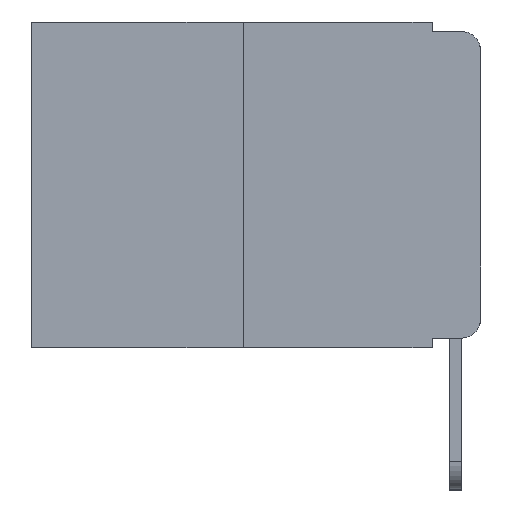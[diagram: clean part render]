
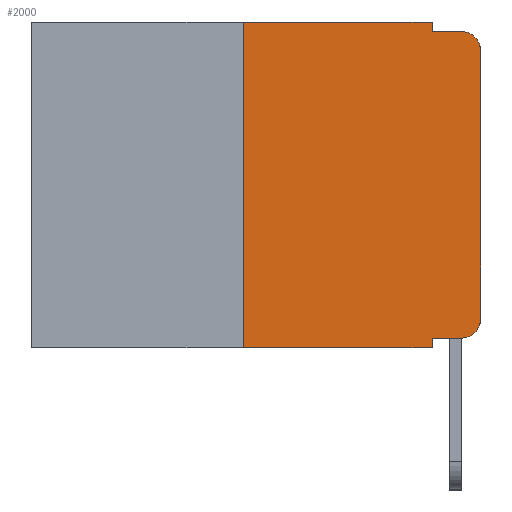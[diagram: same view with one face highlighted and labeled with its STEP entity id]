
A CAD part, left-side view. The second image highlights one B-rep face of the part: STEP entity #2000.
In plain terms, the highlighted planar face has unit normal (-1, 0, 0).
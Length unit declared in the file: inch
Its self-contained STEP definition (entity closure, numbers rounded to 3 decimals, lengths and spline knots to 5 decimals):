
#30 = FACE_OUTER_BOUND ( 'NONE', #903, .T. ) ;
#32 = EDGE_CURVE ( 'NONE', #7247, #2983, #8644, .T. ) ;
#239 = LINE ( 'NONE', #11429, #5632 ) ;
#250 = AXIS2_PLACEMENT_3D ( 'NONE', #5185, #4785, #8455 ) ;
#743 = CARTESIAN_POINT ( 'NONE',  ( 0., 0.051, 0. ) ) ;
#797 = CARTESIAN_POINT ( 'NONE',  ( 0., 0.25, 0. ) ) ;
#903 = EDGE_LOOP ( 'NONE', ( #8469, #4815, #4759, #4670, #4480, #4424, #4358, #4037, #3895, #3824 ) ) ;
#1348 = CARTESIAN_POINT ( 'NONE',  ( 0., 0., -0.03 ) ) ;
#1365 = CARTESIAN_POINT ( 'NONE',  ( 0., 0.051, -0.343 ) ) ;
#1489 = EDGE_CURVE ( 'NONE', #8368, #1525, #239, .T. ) ;
#1525 = VERTEX_POINT ( 'NONE', #1365 ) ;
#1577 = EDGE_CURVE ( 'NONE', #8368, #5704, #2273, .T. ) ;
#1839 = EDGE_CURVE ( 'NONE', #5704, #11722, #10260, .T. ) ;
#1909 = VECTOR ( 'NONE', #2441, 39.37008 ) ;
#1931 = DIRECTION ( 'NONE',  ( 0., 0., 1. ) ) ;
#1970 = CARTESIAN_POINT ( 'NONE',  ( 0., 0.051, -0.333 ) ) ;
#2000 = ADVANCED_FACE ( 'NONE', ( #30 ), #6648, .F. ) ;
#2273 = LINE ( 'NONE', #1970, #9714 ) ;
#2441 = DIRECTION ( 'NONE',  ( 0., -1., 0. ) ) ;
#2983 = VERTEX_POINT ( 'NONE', #10636 ) ;
#3414 = CARTESIAN_POINT ( 'NONE',  ( 0., 0.02, -0.313 ) ) ;
#3684 = CIRCLE ( 'NONE', #7859, 0.02 ) ;
#3748 = DIRECTION ( 'NONE',  ( 0., 0., 1. ) ) ;
#3788 = CARTESIAN_POINT ( 'NONE',  ( 0., 0.02, -0.03 ) ) ;
#3824 = ORIENTED_EDGE ( 'NONE', *, *, #1839, .T. ) ;
#3895 = ORIENTED_EDGE ( 'NONE', *, *, #1577, .T. ) ;
#4037 = ORIENTED_EDGE ( 'NONE', *, *, #1489, .F. ) ;
#4207 = VECTOR ( 'NONE', #6423, 39.37008 ) ;
#4358 = ORIENTED_EDGE ( 'NONE', *, *, #11394, .T. ) ;
#4424 = ORIENTED_EDGE ( 'NONE', *, *, #32, .F. ) ;
#4480 = ORIENTED_EDGE ( 'NONE', *, *, #7723, .F. ) ;
#4621 = VERTEX_POINT ( 'NONE', #8294 ) ;
#4670 = ORIENTED_EDGE ( 'NONE', *, *, #11001, .F. ) ;
#4698 = LINE ( 'NONE', #9266, #1909 ) ;
#4759 = ORIENTED_EDGE ( 'NONE', *, *, #10922, .F. ) ;
#4778 = DIRECTION ( 'NONE',  ( 0., 0., -1. ) ) ;
#4785 = DIRECTION ( 'NONE',  ( 1., 0., 0. ) ) ;
#4815 = ORIENTED_EDGE ( 'NONE', *, *, #10865, .T. ) ;
#4828 = CARTESIAN_POINT ( 'NONE',  ( 0., 0.051, -0.01 ) ) ;
#4966 = VERTEX_POINT ( 'NONE', #11161 ) ;
#5185 = CARTESIAN_POINT ( 'NONE',  ( 0., 0.473, 0. ) ) ;
#5580 = AXIS2_PLACEMENT_3D ( 'NONE', #3414, #6360, #10184 ) ;
#5632 = VECTOR ( 'NONE', #8456, 39.37008 ) ;
#5704 = VERTEX_POINT ( 'NONE', #12509 ) ;
#6018 = LINE ( 'NONE', #4828, #10855 ) ;
#6133 = VECTOR ( 'NONE', #1931, 39.37008 ) ;
#6360 = DIRECTION ( 'NONE',  ( -1., 0., 0. ) ) ;
#6423 = DIRECTION ( 'NONE',  ( 0., -1., 0. ) ) ;
#6583 = LINE ( 'NONE', #10343, #11357 ) ;
#6648 = PLANE ( 'NONE',  #250 ) ;
#6775 = LINE ( 'NONE', #7334, #4207 ) ;
#7021 = DIRECTION ( 'NONE',  ( 0., 0., -1. ) ) ;
#7247 = VERTEX_POINT ( 'NONE', #11215 ) ;
#7334 = CARTESIAN_POINT ( 'NONE',  ( 0., 0.473, -0.343 ) ) ;
#7723 = EDGE_CURVE ( 'NONE', #2983, #4621, #4698, .T. ) ;
#7739 = VERTEX_POINT ( 'NONE', #1348 ) ;
#7859 = AXIS2_PLACEMENT_3D ( 'NONE', #3788, #10387, #4778 ) ;
#7893 = CARTESIAN_POINT ( 'NONE',  ( 0., 0., -0.313 ) ) ;
#8294 = CARTESIAN_POINT ( 'NONE',  ( 0., 0.051, 0. ) ) ;
#8368 = VERTEX_POINT ( 'NONE', #8981 ) ;
#8455 = DIRECTION ( 'NONE',  ( 0., 0., -1. ) ) ;
#8456 = DIRECTION ( 'NONE',  ( 0., 0., -1. ) ) ;
#8469 = ORIENTED_EDGE ( 'NONE', *, *, #10851, .T. ) ;
#8644 = LINE ( 'NONE', #797, #6133 ) ;
#8981 = CARTESIAN_POINT ( 'NONE',  ( 0., 0.051, -0.333 ) ) ;
#9069 = VERTEX_POINT ( 'NONE', #10941 ) ;
#9266 = CARTESIAN_POINT ( 'NONE',  ( 0., 0.473, 0. ) ) ;
#9714 = VECTOR ( 'NONE', #9816, 39.37008 ) ;
#9770 = VECTOR ( 'NONE', #7021, 39.37008 ) ;
#9816 = DIRECTION ( 'NONE',  ( 0., -1., 0. ) ) ;
#10184 = DIRECTION ( 'NONE',  ( 0., 0., -1. ) ) ;
#10260 = CIRCLE ( 'NONE', #5580, 0.02 ) ;
#10343 = CARTESIAN_POINT ( 'NONE',  ( 0., 0., 0. ) ) ;
#10387 = DIRECTION ( 'NONE',  ( -1., 0., 0. ) ) ;
#10636 = CARTESIAN_POINT ( 'NONE',  ( 0., 0.25, 0. ) ) ;
#10851 = EDGE_CURVE ( 'NONE', #11722, #7739, #6583, .T. ) ;
#10855 = VECTOR ( 'NONE', #11229, 39.37008 ) ;
#10865 = EDGE_CURVE ( 'NONE', #7739, #9069, #3684, .T. ) ;
#10922 = EDGE_CURVE ( 'NONE', #4966, #9069, #6018, .T. ) ;
#10941 = CARTESIAN_POINT ( 'NONE',  ( 0., 0.02, -0.01 ) ) ;
#11001 = EDGE_CURVE ( 'NONE', #4621, #4966, #12002, .T. ) ;
#11161 = CARTESIAN_POINT ( 'NONE',  ( 0., 0.051, -0.01 ) ) ;
#11215 = CARTESIAN_POINT ( 'NONE',  ( 0., 0.25, -0.343 ) ) ;
#11229 = DIRECTION ( 'NONE',  ( 0., -1., 0. ) ) ;
#11357 = VECTOR ( 'NONE', #3748, 39.37008 ) ;
#11394 = EDGE_CURVE ( 'NONE', #7247, #1525, #6775, .T. ) ;
#11429 = CARTESIAN_POINT ( 'NONE',  ( 0., 0.051, 0. ) ) ;
#11722 = VERTEX_POINT ( 'NONE', #7893 ) ;
#12002 = LINE ( 'NONE', #743, #9770 ) ;
#12509 = CARTESIAN_POINT ( 'NONE',  ( 0., 0.02, -0.333 ) ) ;
